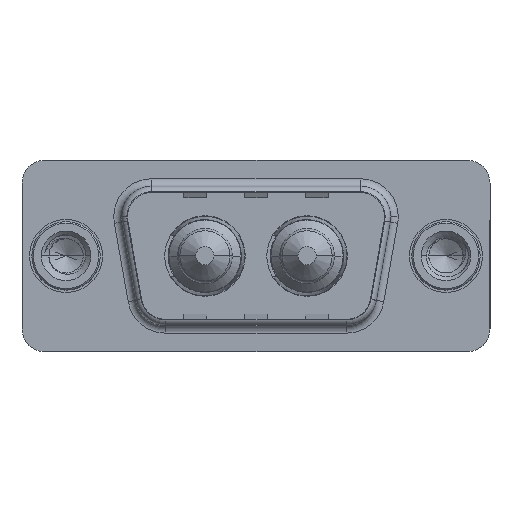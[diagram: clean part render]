
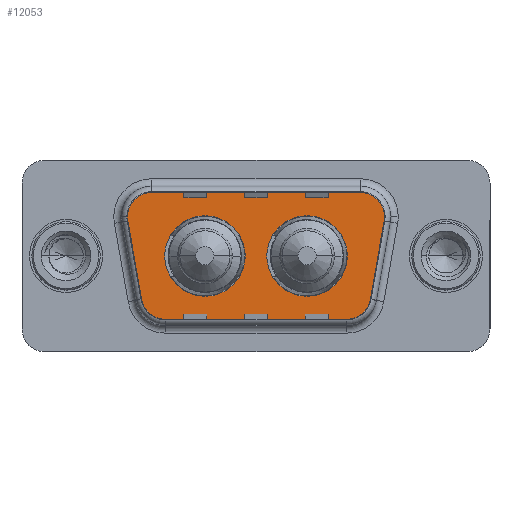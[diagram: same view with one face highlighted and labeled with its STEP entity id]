
A CAD part, top view. The second image highlights one B-rep face of the part: STEP entity #12053.
In plain terms, the highlighted planar face has unit normal (0, 0, 1).
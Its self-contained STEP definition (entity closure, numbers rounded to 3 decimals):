
#78 = CIRCLE ( 'NONE', #8738, 2.65 ) ;
#134 = EDGE_CURVE ( 'NONE', #3294, #16871, #78, .T. ) ;
#288 = ORIENTED_EDGE ( 'NONE', *, *, #17074, .T. ) ;
#521 = EDGE_CURVE ( 'NONE', #5618, #2637, #1713, .T. ) ;
#750 = EDGE_CURVE ( 'NONE', #14293, #5618, #10556, .T. ) ;
#865 = CIRCLE ( 'NONE', #13619, 2.65 ) ;
#1002 = VERTEX_POINT ( 'NONE', #14765 ) ;
#1072 = AXIS2_PLACEMENT_3D ( 'NONE', #2590, #12657, #4055 ) ;
#1148 = DIRECTION ( 'NONE',  ( 1., 0., 0. ) ) ;
#1327 = ORIENTED_EDGE ( 'NONE', *, *, #6899, .T. ) ;
#1349 = ORIENTED_EDGE ( 'NONE', *, *, #750, .T. ) ;
#1617 = AXIS2_PLACEMENT_3D ( 'NONE', #14040, #9828, #1148 ) ;
#1713 = LINE ( 'NONE', #2268, #12331 ) ;
#1735 = CARTESIAN_POINT ( 'NONE',  ( 21.534, 2.553, 0. ) ) ;
#1895 = EDGE_CURVE ( 'NONE', #6581, #7725, #6028, .T. ) ;
#1995 = AXIS2_PLACEMENT_3D ( 'NONE', #17401, #17336, #17277 ) ;
#2193 = AXIS2_PLACEMENT_3D ( 'NONE', #12343, #15155, #8858 ) ;
#2221 = VERTEX_POINT ( 'NONE', #16286 ) ;
#2268 = CARTESIAN_POINT ( 'NONE',  ( 21.534, 2.553, 0. ) ) ;
#2515 = VERTEX_POINT ( 'NONE', #18168 ) ;
#2520 = FACE_BOUND ( 'NONE', #6751, .T. ) ;
#2590 = CARTESIAN_POINT ( 'NONE',  ( 15.86, 0., 0. ) ) ;
#2637 = VERTEX_POINT ( 'NONE', #1735 ) ;
#2639 = VECTOR ( 'NONE', #6927, 1000. ) ;
#2674 = ORIENTED_EDGE ( 'NONE', *, *, #1895, .T. ) ;
#3096 = LINE ( 'NONE', #13970, #2639 ) ;
#3180 = VERTEX_POINT ( 'NONE', #17564 ) ;
#3250 = VERTEX_POINT ( 'NONE', #14593 ) ;
#3294 = VERTEX_POINT ( 'NONE', #6384 ) ;
#3408 = ORIENTED_EDGE ( 'NONE', *, *, #9177, .T. ) ;
#3556 = ORIENTED_EDGE ( 'NONE', *, *, #12938, .T. ) ;
#3778 = EDGE_CURVE ( 'NONE', #3180, #1002, #10707, .T. ) ;
#4055 = DIRECTION ( 'NONE',  ( 1., 0., 0. ) ) ;
#4067 = CARTESIAN_POINT ( 'NONE',  ( 19.564, 2.9, 0. ) ) ;
#4952 = DIRECTION ( 'NONE',  ( 0., 0., 1. ) ) ;
#5335 = ORIENTED_EDGE ( 'NONE', *, *, #521, .T. ) ;
#5516 = CIRCLE ( 'NONE', #1995, 2. ) ;
#5522 = DIRECTION ( 'NONE',  ( 0.174, 0.985, 0. ) ) ;
#5560 = DIRECTION ( 'NONE',  ( -1., 0., 0. ) ) ;
#5563 = EDGE_CURVE ( 'NONE', #2221, #11454, #5516, .T. ) ;
#5618 = VERTEX_POINT ( 'NONE', #11878 ) ;
#5874 = ORIENTED_EDGE ( 'NONE', *, *, #13615, .F. ) ;
#6028 = CIRCLE ( 'NONE', #14993, 2. ) ;
#6054 = CARTESIAN_POINT ( 'NONE',  ( 21.564, 2.9, 0. ) ) ;
#6092 = EDGE_LOOP ( 'NONE', ( #1349, #5335, #3408, #2674, #8971, #17780, #1327, #3556, #288 ) ) ;
#6139 = DIRECTION ( 'NONE',  ( 0., 0., 1. ) ) ;
#6170 = CIRCLE ( 'NONE', #10569, 2. ) ;
#6384 = CARTESIAN_POINT ( 'NONE',  ( 11.79, 0., 0. ) ) ;
#6581 = VERTEX_POINT ( 'NONE', #6054 ) ;
#6751 = EDGE_LOOP ( 'NONE', ( #13222, #5874 ) ) ;
#6899 = EDGE_CURVE ( 'NONE', #11454, #3250, #9254, .T. ) ;
#6927 = DIRECTION ( 'NONE',  ( 1., 0., 0. ) ) ;
#7645 = CARTESIAN_POINT ( 'NONE',  ( 9.14, 0., 0. ) ) ;
#7725 = VERTEX_POINT ( 'NONE', #15908 ) ;
#7797 = CARTESIAN_POINT ( 'NONE',  ( 18.541, -4.9, 0. ) ) ;
#8738 = AXIS2_PLACEMENT_3D ( 'NONE', #10664, #12914, #11792 ) ;
#8770 = CIRCLE ( 'NONE', #1072, 2.65 ) ;
#8858 = DIRECTION ( 'NONE',  ( 1., 0., 0. ) ) ;
#8971 = ORIENTED_EDGE ( 'NONE', *, *, #16023, .T. ) ;
#9094 = DIRECTION ( 'NONE',  ( 1., 0., 0. ) ) ;
#9177 = EDGE_CURVE ( 'NONE', #2637, #6581, #17588, .T. ) ;
#9254 = LINE ( 'NONE', #15325, #16304 ) ;
#9753 = FACE_BOUND ( 'NONE', #14321, .T. ) ;
#9828 = DIRECTION ( 'NONE',  ( 0., 0., 1. ) ) ;
#10053 = ORIENTED_EDGE ( 'NONE', *, *, #3778, .F. ) ;
#10195 = FACE_OUTER_BOUND ( 'NONE', #6092, .T. ) ;
#10281 = CARTESIAN_POINT ( 'NONE',  ( 19.564, 2.9, 0. ) ) ;
#10556 = CIRCLE ( 'NONE', #2193, 2. ) ;
#10569 = AXIS2_PLACEMENT_3D ( 'NONE', #14606, #6139, #16040 ) ;
#10602 = VECTOR ( 'NONE', #14344, 1000. ) ;
#10664 = CARTESIAN_POINT ( 'NONE',  ( 9.14, 0., 0. ) ) ;
#10707 = CIRCLE ( 'NONE', #12896, 2.65 ) ;
#11263 = CARTESIAN_POINT ( 'NONE',  ( 6.49, 0., 0. ) ) ;
#11454 = VERTEX_POINT ( 'NONE', #15709 ) ;
#11558 = CARTESIAN_POINT ( 'NONE',  ( 5.436, 4.9, 0. ) ) ;
#11792 = DIRECTION ( 'NONE',  ( 1., 0., 0. ) ) ;
#11878 = CARTESIAN_POINT ( 'NONE',  ( 20.511, -3.247, 0. ) ) ;
#11908 = ORIENTED_EDGE ( 'NONE', *, *, #16859, .F. ) ;
#12053 = ADVANCED_FACE ( 'NONE', ( #9753, #2520, #10195 ), #18318, .T. ) ;
#12331 = VECTOR ( 'NONE', #5522, 1000. ) ;
#12343 = CARTESIAN_POINT ( 'NONE',  ( 18.541, -2.9, 0. ) ) ;
#12351 = AXIS2_PLACEMENT_3D ( 'NONE', #4067, #14070, #5560 ) ;
#12657 = DIRECTION ( 'NONE',  ( 0., 0., 1. ) ) ;
#12896 = AXIS2_PLACEMENT_3D ( 'NONE', #16997, #16922, #13766 ) ;
#12914 = DIRECTION ( 'NONE',  ( 0., 0., 1. ) ) ;
#12938 = EDGE_CURVE ( 'NONE', #3250, #2515, #6170, .T. ) ;
#13222 = ORIENTED_EDGE ( 'NONE', *, *, #134, .F. ) ;
#13615 = EDGE_CURVE ( 'NONE', #16871, #3294, #865, .T. ) ;
#13619 = AXIS2_PLACEMENT_3D ( 'NONE', #7645, #17559, #9094 ) ;
#13766 = DIRECTION ( 'NONE',  ( 1., 0., 0. ) ) ;
#13970 = CARTESIAN_POINT ( 'NONE',  ( 6.459, -4.9, 0. ) ) ;
#14040 = CARTESIAN_POINT ( 'NONE',  ( 18.541, -2.9, 0. ) ) ;
#14070 = DIRECTION ( 'NONE',  ( 0., 0., 1. ) ) ;
#14293 = VERTEX_POINT ( 'NONE', #7797 ) ;
#14321 = EDGE_LOOP ( 'NONE', ( #11908, #10053 ) ) ;
#14344 = DIRECTION ( 'NONE',  ( -1., 0., 0. ) ) ;
#14593 = CARTESIAN_POINT ( 'NONE',  ( 4.489, -3.247, 0. ) ) ;
#14606 = CARTESIAN_POINT ( 'NONE',  ( 6.459, -2.9, 0. ) ) ;
#14765 = CARTESIAN_POINT ( 'NONE',  ( 18.51, 0., 0. ) ) ;
#14993 = AXIS2_PLACEMENT_3D ( 'NONE', #10281, #4952, #15840 ) ;
#15155 = DIRECTION ( 'NONE',  ( 0., 0., 1. ) ) ;
#15325 = CARTESIAN_POINT ( 'NONE',  ( 3.466, 2.553, 0. ) ) ;
#15379 = DIRECTION ( 'NONE',  ( 0.174, -0.985, 0. ) ) ;
#15709 = CARTESIAN_POINT ( 'NONE',  ( 3.466, 2.553, 0. ) ) ;
#15840 = DIRECTION ( 'NONE',  ( -1., 0., 0. ) ) ;
#15908 = CARTESIAN_POINT ( 'NONE',  ( 19.564, 4.9, 0. ) ) ;
#16023 = EDGE_CURVE ( 'NONE', #7725, #2221, #18541, .T. ) ;
#16040 = DIRECTION ( 'NONE',  ( -1., 0., 0. ) ) ;
#16286 = CARTESIAN_POINT ( 'NONE',  ( 5.436, 4.9, 0. ) ) ;
#16304 = VECTOR ( 'NONE', #15379, 1000. ) ;
#16859 = EDGE_CURVE ( 'NONE', #1002, #3180, #8770, .T. ) ;
#16871 = VERTEX_POINT ( 'NONE', #11263 ) ;
#16922 = DIRECTION ( 'NONE',  ( 0., 0., 1. ) ) ;
#16997 = CARTESIAN_POINT ( 'NONE',  ( 15.86, 0., 0. ) ) ;
#17074 = EDGE_CURVE ( 'NONE', #2515, #14293, #3096, .T. ) ;
#17277 = DIRECTION ( 'NONE',  ( 1., 0., 0. ) ) ;
#17336 = DIRECTION ( 'NONE',  ( 0., 0., 1. ) ) ;
#17401 = CARTESIAN_POINT ( 'NONE',  ( 5.436, 2.9, 0. ) ) ;
#17559 = DIRECTION ( 'NONE',  ( 0., 0., 1. ) ) ;
#17564 = CARTESIAN_POINT ( 'NONE',  ( 13.21, 0., 0. ) ) ;
#17588 = CIRCLE ( 'NONE', #12351, 2. ) ;
#17780 = ORIENTED_EDGE ( 'NONE', *, *, #5563, .T. ) ;
#18168 = CARTESIAN_POINT ( 'NONE',  ( 6.459, -4.9, 0. ) ) ;
#18318 = PLANE ( 'NONE',  #1617 ) ;
#18541 = LINE ( 'NONE', #11558, #10602 ) ;
